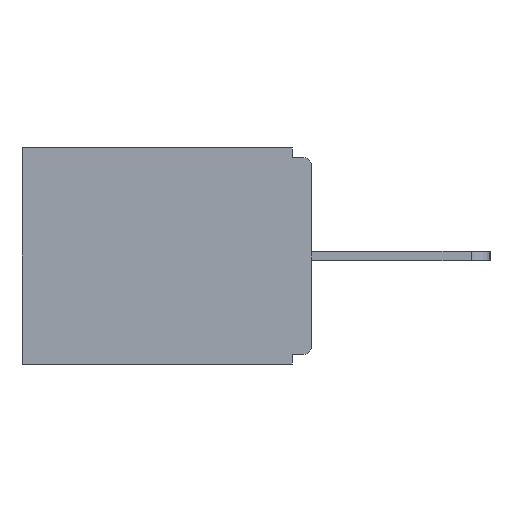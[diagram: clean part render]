
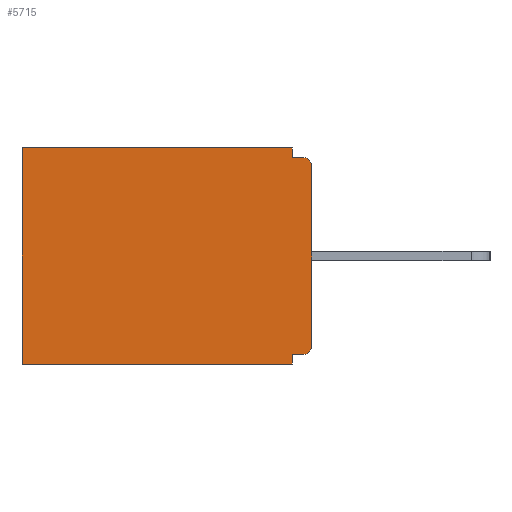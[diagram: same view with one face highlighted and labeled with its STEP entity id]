
A CAD part, left-side view. The second image highlights one B-rep face of the part: STEP entity #5715.
In plain terms, the highlighted planar face has unit normal (-1, 0, 0).
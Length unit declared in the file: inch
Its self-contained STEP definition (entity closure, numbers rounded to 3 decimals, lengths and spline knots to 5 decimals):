
#346 = VERTEX_POINT ( 'NONE', #4907 ) ;
#386 = DIRECTION ( 'NONE',  ( 0., 0., -1. ) ) ;
#685 = ORIENTED_EDGE ( 'NONE', *, *, #9519, .T. ) ;
#718 = DIRECTION ( 'NONE',  ( 0., 1., 0. ) ) ;
#932 = VECTOR ( 'NONE', #7389, 39.37008 ) ;
#1012 = ORIENTED_EDGE ( 'NONE', *, *, #15097, .T. ) ;
#1298 = CIRCLE ( 'NONE', #5117, 0.015 ) ;
#1385 = CARTESIAN_POINT ( 'NONE',  ( 0.298, 0., 0. ) ) ;
#1532 = VECTOR ( 'NONE', #4389, 39.37008 ) ;
#1700 = EDGE_CURVE ( 'NONE', #3585, #8623, #6724, .T. ) ;
#2143 = DIRECTION ( 'NONE',  ( 0., 0., -1. ) ) ;
#2313 = CARTESIAN_POINT ( 'NONE',  ( 0.298, 0.031, -0.343 ) ) ;
#2683 = LINE ( 'NONE', #14690, #3200 ) ;
#2799 = LINE ( 'NONE', #15298, #932 ) ;
#2960 = VECTOR ( 'NONE', #386, 39.37008 ) ;
#3046 = ORIENTED_EDGE ( 'NONE', *, *, #9878, .F. ) ;
#3078 = EDGE_CURVE ( 'NONE', #6541, #8163, #1298, .T. ) ;
#3200 = VECTOR ( 'NONE', #7086, 39.37008 ) ;
#3585 = VERTEX_POINT ( 'NONE', #2313 ) ;
#4131 = CARTESIAN_POINT ( 'NONE',  ( 0.298, 0., -0.03 ) ) ;
#4155 = DIRECTION ( 'NONE',  ( 0., 0., -1. ) ) ;
#4389 = DIRECTION ( 'NONE',  ( 0., 1., 0. ) ) ;
#4816 = VECTOR ( 'NONE', #718, 39.37008 ) ;
#4876 = VERTEX_POINT ( 'NONE', #11714 ) ;
#4907 = CARTESIAN_POINT ( 'NONE',  ( 0.298, 0.031, 0. ) ) ;
#5117 = AXIS2_PLACEMENT_3D ( 'NONE', #11221, #15736, #14322 ) ;
#5408 = AXIS2_PLACEMENT_3D ( 'NONE', #10516, #5632, #4155 ) ;
#5512 = CARTESIAN_POINT ( 'NONE',  ( 0.298, 0.031, -0.328 ) ) ;
#5632 = DIRECTION ( 'NONE',  ( 1., 0., 0. ) ) ;
#5715 = ADVANCED_FACE ( 'NONE', ( #19541 ), #16443, .F. ) ;
#5876 = LINE ( 'NONE', #1385, #1532 ) ;
#6039 = EDGE_CURVE ( 'NONE', #9364, #3585, #2683, .T. ) ;
#6541 = VERTEX_POINT ( 'NONE', #18915 ) ;
#6596 = DIRECTION ( 'NONE',  ( 0., 0., -1. ) ) ;
#6700 = CARTESIAN_POINT ( 'NONE',  ( 0.298, 0.015, -0.03 ) ) ;
#6724 = LINE ( 'NONE', #7016, #4816 ) ;
#6784 = DIRECTION ( 'NONE',  ( 0., 1., 0. ) ) ;
#7016 = CARTESIAN_POINT ( 'NONE',  ( 0.298, 0., -0.343 ) ) ;
#7086 = DIRECTION ( 'NONE',  ( 0., 0., -1. ) ) ;
#7389 = DIRECTION ( 'NONE',  ( 0., 0., -1. ) ) ;
#7543 = LINE ( 'NONE', #14965, #10743 ) ;
#7544 = EDGE_LOOP ( 'NONE', ( #18502, #19175, #16026, #1012, #685, #10226, #11011, #8958, #16557, #3046 ) ) ;
#8163 = VERTEX_POINT ( 'NONE', #16909 ) ;
#8361 = EDGE_CURVE ( 'NONE', #15898, #12151, #19514, .T. ) ;
#8623 = VERTEX_POINT ( 'NONE', #8770 ) ;
#8770 = CARTESIAN_POINT ( 'NONE',  ( 0.298, 0.46, -0.343 ) ) ;
#8787 = VERTEX_POINT ( 'NONE', #14283 ) ;
#8958 = ORIENTED_EDGE ( 'NONE', *, *, #15352, .F. ) ;
#9364 = VERTEX_POINT ( 'NONE', #5512 ) ;
#9519 = EDGE_CURVE ( 'NONE', #4876, #8623, #11399, .T. ) ;
#9878 = EDGE_CURVE ( 'NONE', #15898, #8163, #2799, .T. ) ;
#10132 = VECTOR ( 'NONE', #2143, 39.37008 ) ;
#10226 = ORIENTED_EDGE ( 'NONE', *, *, #1700, .F. ) ;
#10516 = CARTESIAN_POINT ( 'NONE',  ( 0.298, 0., 0. ) ) ;
#10633 = DIRECTION ( 'NONE',  ( 0., -1., 0. ) ) ;
#10743 = VECTOR ( 'NONE', #10633, 39.37008 ) ;
#11011 = ORIENTED_EDGE ( 'NONE', *, *, #6039, .F. ) ;
#11221 = CARTESIAN_POINT ( 'NONE',  ( 0.298, 0.015, -0.313 ) ) ;
#11285 = CARTESIAN_POINT ( 'NONE',  ( 0.298, 0., -0.328 ) ) ;
#11399 = LINE ( 'NONE', #17210, #2960 ) ;
#11714 = CARTESIAN_POINT ( 'NONE',  ( 0.298, 0.46, 0. ) ) ;
#12151 = VERTEX_POINT ( 'NONE', #13381 ) ;
#13232 = CARTESIAN_POINT ( 'NONE',  ( 0.298, 0.031, -0.343 ) ) ;
#13381 = CARTESIAN_POINT ( 'NONE',  ( 0.298, 0.015, -0.015 ) ) ;
#13779 = EDGE_CURVE ( 'NONE', #8787, #12151, #7543, .T. ) ;
#14283 = CARTESIAN_POINT ( 'NONE',  ( 0.298, 0.031, -0.015 ) ) ;
#14322 = DIRECTION ( 'NONE',  ( 0., 0., -1. ) ) ;
#14387 = LINE ( 'NONE', #11285, #15200 ) ;
#14413 = AXIS2_PLACEMENT_3D ( 'NONE', #6700, #15610, #6596 ) ;
#14532 = LINE ( 'NONE', #13232, #10132 ) ;
#14690 = CARTESIAN_POINT ( 'NONE',  ( 0.298, 0.031, -0.343 ) ) ;
#14965 = CARTESIAN_POINT ( 'NONE',  ( 0.298, 0., -0.015 ) ) ;
#15097 = EDGE_CURVE ( 'NONE', #346, #4876, #5876, .T. ) ;
#15200 = VECTOR ( 'NONE', #6784, 39.37008 ) ;
#15298 = CARTESIAN_POINT ( 'NONE',  ( 0.298, 0., 0. ) ) ;
#15352 = EDGE_CURVE ( 'NONE', #6541, #9364, #14387, .T. ) ;
#15610 = DIRECTION ( 'NONE',  ( -1., 0., 0. ) ) ;
#15736 = DIRECTION ( 'NONE',  ( -1., 0., 0. ) ) ;
#15898 = VERTEX_POINT ( 'NONE', #4131 ) ;
#16026 = ORIENTED_EDGE ( 'NONE', *, *, #19217, .F. ) ;
#16443 = PLANE ( 'NONE',  #5408 ) ;
#16557 = ORIENTED_EDGE ( 'NONE', *, *, #3078, .T. ) ;
#16909 = CARTESIAN_POINT ( 'NONE',  ( 0.298, 0., -0.313 ) ) ;
#17210 = CARTESIAN_POINT ( 'NONE',  ( 0.298, 0.46, 0. ) ) ;
#18502 = ORIENTED_EDGE ( 'NONE', *, *, #8361, .T. ) ;
#18915 = CARTESIAN_POINT ( 'NONE',  ( 0.298, 0.015, -0.328 ) ) ;
#19175 = ORIENTED_EDGE ( 'NONE', *, *, #13779, .F. ) ;
#19217 = EDGE_CURVE ( 'NONE', #346, #8787, #14532, .T. ) ;
#19514 = CIRCLE ( 'NONE', #14413, 0.015 ) ;
#19541 = FACE_OUTER_BOUND ( 'NONE', #7544, .T. ) ;
